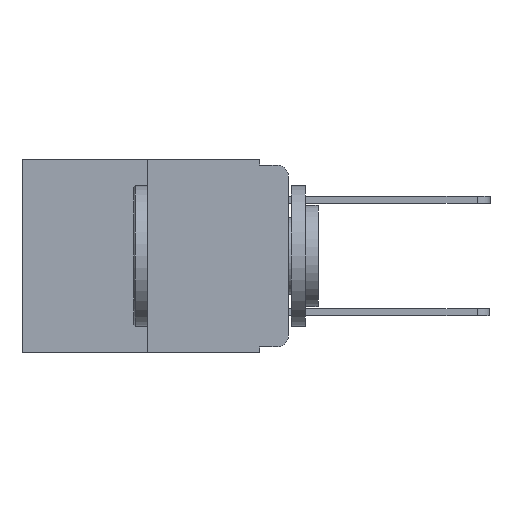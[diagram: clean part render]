
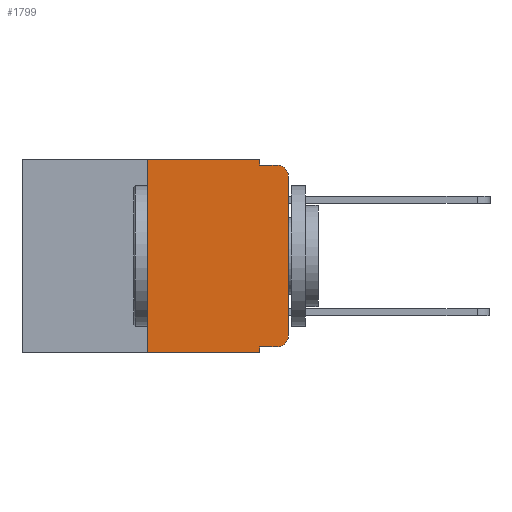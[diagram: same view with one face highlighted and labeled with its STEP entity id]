
A CAD part, left-side view. The second image highlights one B-rep face of the part: STEP entity #1799.
In plain terms, the highlighted planar face has unit normal (-1, 0, 0).
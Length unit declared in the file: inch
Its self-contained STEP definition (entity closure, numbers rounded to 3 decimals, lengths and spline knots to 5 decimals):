
#194 = ORIENTED_EDGE ( 'NONE', *, *, #15623, .F. ) ;
#346 = AXIS2_PLACEMENT_3D ( 'NONE', #11494, #17820, #3595 ) ;
#868 = VECTOR ( 'NONE', #3230, 39.37008 ) ;
#911 = FACE_OUTER_BOUND ( 'NONE', #3137, .T. ) ;
#994 = ORIENTED_EDGE ( 'NONE', *, *, #17917, .T. ) ;
#1089 = CIRCLE ( 'NONE', #3722, 0.02 ) ;
#1510 = PLANE ( 'NONE',  #346 ) ;
#1540 = CARTESIAN_POINT ( 'NONE',  ( 0., 0.473, 0. ) ) ;
#1620 = VECTOR ( 'NONE', #2763, 39.37008 ) ;
#1716 = LINE ( 'NONE', #19185, #8344 ) ;
#1799 = ADVANCED_FACE ( 'NONE', ( #911 ), #1510, .F. ) ;
#2071 = DIRECTION ( 'NONE',  ( 0., 0., -1. ) ) ;
#2132 = CARTESIAN_POINT ( 'NONE',  ( 0., 0.02, -0.03 ) ) ;
#2307 = ORIENTED_EDGE ( 'NONE', *, *, #9351, .T. ) ;
#2413 = VECTOR ( 'NONE', #4433, 39.37008 ) ;
#2444 = CARTESIAN_POINT ( 'NONE',  ( 0., 0.25, -0.343 ) ) ;
#2655 = CIRCLE ( 'NONE', #17033, 0.02 ) ;
#2763 = DIRECTION ( 'NONE',  ( 0., -1., 0. ) ) ;
#2993 = CARTESIAN_POINT ( 'NONE',  ( 0., 0.02, -0.333 ) ) ;
#3137 = EDGE_LOOP ( 'NONE', ( #11713, #994, #13979, #3593, #194, #6250, #2307, #15955, #9168, #10570 ) ) ;
#3230 = DIRECTION ( 'NONE',  ( 0., -1., 0. ) ) ;
#3593 = ORIENTED_EDGE ( 'NONE', *, *, #13913, .F. ) ;
#3595 = DIRECTION ( 'NONE',  ( 0., 0., -1. ) ) ;
#3722 = AXIS2_PLACEMENT_3D ( 'NONE', #2132, #13074, #3805 ) ;
#3805 = DIRECTION ( 'NONE',  ( 0., 0., -1. ) ) ;
#3885 = VERTEX_POINT ( 'NONE', #2993 ) ;
#3989 = DIRECTION ( 'NONE',  ( 0., 0., -1. ) ) ;
#4020 = DIRECTION ( 'NONE',  ( -1., 0., 0. ) ) ;
#4039 = CARTESIAN_POINT ( 'NONE',  ( 0., 0.02, -0.313 ) ) ;
#4046 = CARTESIAN_POINT ( 'NONE',  ( 0., 0.051, -0.343 ) ) ;
#4123 = VERTEX_POINT ( 'NONE', #11721 ) ;
#4332 = EDGE_CURVE ( 'NONE', #3885, #18530, #2655, .T. ) ;
#4433 = DIRECTION ( 'NONE',  ( 0., -1., 0. ) ) ;
#4674 = CARTESIAN_POINT ( 'NONE',  ( 0., 0.051, 0. ) ) ;
#4825 = LINE ( 'NONE', #1540, #868 ) ;
#5415 = EDGE_CURVE ( 'NONE', #4123, #8513, #6094, .T. ) ;
#5480 = VERTEX_POINT ( 'NONE', #9117 ) ;
#5553 = VECTOR ( 'NONE', #19250, 39.37008 ) ;
#5914 = CARTESIAN_POINT ( 'NONE',  ( 0., 0.051, 0. ) ) ;
#6094 = LINE ( 'NONE', #5914, #10171 ) ;
#6250 = ORIENTED_EDGE ( 'NONE', *, *, #11958, .F. ) ;
#7698 = CARTESIAN_POINT ( 'NONE',  ( 0., 0.051, -0.333 ) ) ;
#7786 = CARTESIAN_POINT ( 'NONE',  ( 0., 0.25, 0. ) ) ;
#8344 = VECTOR ( 'NONE', #12258, 39.37008 ) ;
#8513 = VERTEX_POINT ( 'NONE', #4046 ) ;
#9117 = CARTESIAN_POINT ( 'NONE',  ( 0., 0., -0.03 ) ) ;
#9168 = ORIENTED_EDGE ( 'NONE', *, *, #16250, .T. ) ;
#9181 = CARTESIAN_POINT ( 'NONE',  ( 0., 0.473, -0.343 ) ) ;
#9351 = EDGE_CURVE ( 'NONE', #19362, #8513, #19517, .T. ) ;
#9694 = LINE ( 'NONE', #7786, #5553 ) ;
#9881 = VERTEX_POINT ( 'NONE', #14961 ) ;
#9981 = EDGE_CURVE ( 'NONE', #18530, #5480, #1716, .T. ) ;
#10039 = CARTESIAN_POINT ( 'NONE',  ( 0., 0., -0.313 ) ) ;
#10171 = VECTOR ( 'NONE', #16243, 39.37008 ) ;
#10570 = ORIENTED_EDGE ( 'NONE', *, *, #4332, .T. ) ;
#10694 = DIRECTION ( 'NONE',  ( 0., -1., 0. ) ) ;
#11494 = CARTESIAN_POINT ( 'NONE',  ( 0., 0.473, 0. ) ) ;
#11591 = CARTESIAN_POINT ( 'NONE',  ( 0., 0.051, 0. ) ) ;
#11713 = ORIENTED_EDGE ( 'NONE', *, *, #9981, .T. ) ;
#11721 = CARTESIAN_POINT ( 'NONE',  ( 0., 0.051, -0.333 ) ) ;
#11958 = EDGE_CURVE ( 'NONE', #19362, #17808, #9694, .T. ) ;
#12131 = VECTOR ( 'NONE', #10694, 39.37008 ) ;
#12258 = DIRECTION ( 'NONE',  ( 0., 0., 1. ) ) ;
#12767 = CARTESIAN_POINT ( 'NONE',  ( 0., 0.25, 0. ) ) ;
#13074 = DIRECTION ( 'NONE',  ( -1., 0., 0. ) ) ;
#13496 = LINE ( 'NONE', #11591, #13943 ) ;
#13911 = CARTESIAN_POINT ( 'NONE',  ( 0., 0.02, -0.01 ) ) ;
#13913 = EDGE_CURVE ( 'NONE', #14854, #9881, #13496, .T. ) ;
#13943 = VECTOR ( 'NONE', #2071, 39.37008 ) ;
#13979 = ORIENTED_EDGE ( 'NONE', *, *, #17597, .F. ) ;
#14730 = LINE ( 'NONE', #16386, #2413 ) ;
#14854 = VERTEX_POINT ( 'NONE', #4674 ) ;
#14961 = CARTESIAN_POINT ( 'NONE',  ( 0., 0.051, -0.01 ) ) ;
#15555 = VERTEX_POINT ( 'NONE', #13911 ) ;
#15623 = EDGE_CURVE ( 'NONE', #17808, #14854, #4825, .T. ) ;
#15955 = ORIENTED_EDGE ( 'NONE', *, *, #5415, .F. ) ;
#16243 = DIRECTION ( 'NONE',  ( 0., 0., -1. ) ) ;
#16250 = EDGE_CURVE ( 'NONE', #4123, #3885, #17693, .T. ) ;
#16386 = CARTESIAN_POINT ( 'NONE',  ( 0., 0.051, -0.01 ) ) ;
#17033 = AXIS2_PLACEMENT_3D ( 'NONE', #4039, #4020, #3989 ) ;
#17597 = EDGE_CURVE ( 'NONE', #9881, #15555, #14730, .T. ) ;
#17693 = LINE ( 'NONE', #7698, #1620 ) ;
#17808 = VERTEX_POINT ( 'NONE', #12767 ) ;
#17820 = DIRECTION ( 'NONE',  ( 1., 0., 0. ) ) ;
#17917 = EDGE_CURVE ( 'NONE', #5480, #15555, #1089, .T. ) ;
#18530 = VERTEX_POINT ( 'NONE', #10039 ) ;
#19185 = CARTESIAN_POINT ( 'NONE',  ( 0., 0., 0. ) ) ;
#19250 = DIRECTION ( 'NONE',  ( 0., 0., 1. ) ) ;
#19362 = VERTEX_POINT ( 'NONE', #2444 ) ;
#19517 = LINE ( 'NONE', #9181, #12131 ) ;
